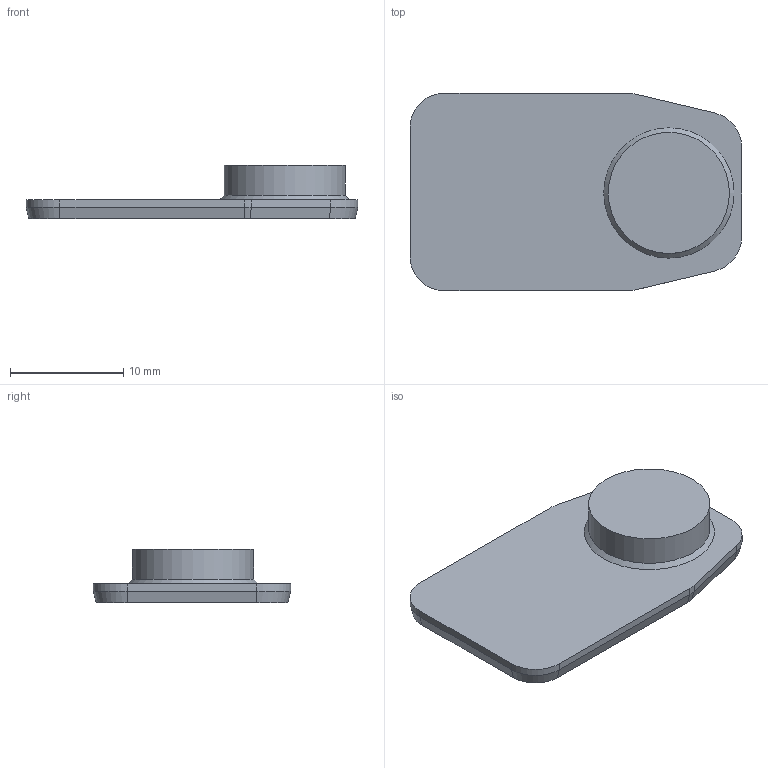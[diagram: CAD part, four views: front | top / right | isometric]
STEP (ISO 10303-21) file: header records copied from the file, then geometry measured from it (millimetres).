
FILE_DESCRIPTION(/* description */ (''),/* implementation_level */ '2;1');
FILE_NAME(/* name */ 'T-Mag Locking Tab v1.step',/* time_stamp */ '2022-06-30T09:14:16-05:00',/* author */ (''),/* organization */ (''),/* preprocessor_version */ 'ST-DEVELOPER v19',/* originating_system */ 'Autodesk Translation Framework v11.7.0.108',/* authorisation */ '');
FILE_SCHEMA (('AUTOMOTIVE_DESIGN { 1 0 10303 214 3 1 1 }'));
Length unit declared in the file: millimetre
Products named in the file (1): Locking Tab Standard v2.0
Bounding box: 29.36 x 17.47 x 4.7 mm (x, y, z)
Volume: 1066 mm3; surface area: 1184.4 mm2
Topology: 1 solids, 1 shells, 29 faces, 65 edges, 39 vertices
Faces by surface type: plane 15, cone 7, cylinder 7
Full cylindrical faces by diameter (mm): 10.719 x1
Entity records: 836 total; most frequent: DIRECTION 146, CARTESIAN_POINT 134, ORIENTED_EDGE 130, EDGE_CURVE 65, AXIS2_PLACEMENT_3D 51, LINE 44, VECTOR 44, VERTEX_POINT 39
